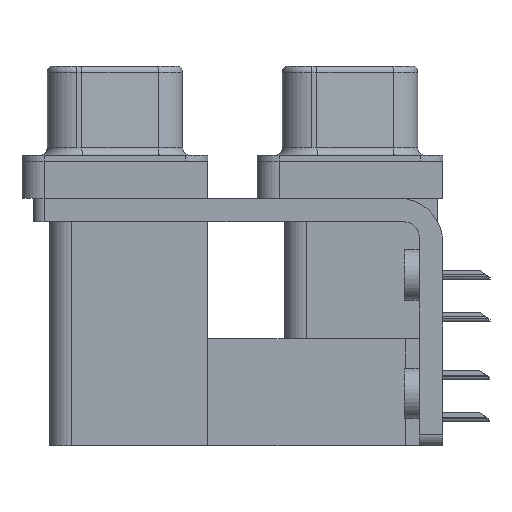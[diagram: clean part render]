
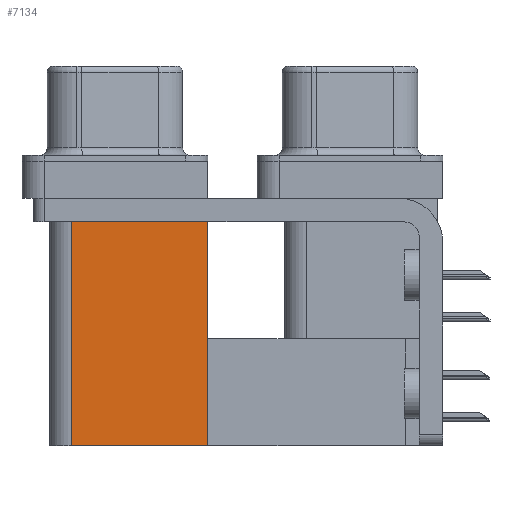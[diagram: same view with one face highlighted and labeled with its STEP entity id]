
A CAD part, left-side view. The second image highlights one B-rep face of the part: STEP entity #7134.
In plain terms, the highlighted planar face has unit normal (-1, 0, 0).
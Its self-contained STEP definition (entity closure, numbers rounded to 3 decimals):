
#318 = EDGE_CURVE ( 'NONE', #9091, #7233, #33261, .T. ) ;
#2637 = CARTESIAN_POINT ( 'NONE',  ( 3.7, 9.6, -2.5 ) ) ;
#3013 = DIRECTION ( 'NONE',  ( 0., 0., 1. ) ) ;
#3194 = EDGE_CURVE ( 'NONE', #9091, #11951, #14326, .T. ) ;
#3592 = DIRECTION ( 'NONE',  ( 0., 1., 0. ) ) ;
#4525 = ORIENTED_EDGE ( 'NONE', *, *, #318, .F. ) ;
#5223 = EDGE_CURVE ( 'NONE', #7233, #37571, #37001, .T. ) ;
#5341 = FACE_OUTER_BOUND ( 'NONE', #20716, .T. ) ;
#6161 = EDGE_CURVE ( 'NONE', #11951, #37571, #36042, .T. ) ;
#6787 = DIRECTION ( 'NONE',  ( 0., 1., 0. ) ) ;
#7134 = ADVANCED_FACE ( 'NONE', ( #5341 ), #27677, .F. ) ;
#7233 = VERTEX_POINT ( 'NONE', #25068 ) ;
#7325 = CARTESIAN_POINT ( 'NONE',  ( 3.7, 18.8, -19.2 ) ) ;
#8796 = DIRECTION ( 'NONE',  ( 0., 0., -1. ) ) ;
#9091 = VERTEX_POINT ( 'NONE', #31145 ) ;
#11951 = VERTEX_POINT ( 'NONE', #2637 ) ;
#12646 = CARTESIAN_POINT ( 'NONE',  ( 3.7, 9.6, -2.5 ) ) ;
#14326 = LINE ( 'NONE', #27563, #18866 ) ;
#15323 = ORIENTED_EDGE ( 'NONE', *, *, #3194, .T. ) ;
#17691 = CARTESIAN_POINT ( 'NONE',  ( 3.7, 18.8, -2.5 ) ) ;
#18103 = DIRECTION ( 'NONE',  ( 1., 0., 0. ) ) ;
#18866 = VECTOR ( 'NONE', #40767, 1000. ) ;
#20716 = EDGE_LOOP ( 'NONE', ( #32661, #38768, #4525, #15323 ) ) ;
#25068 = CARTESIAN_POINT ( 'NONE',  ( 3.7, 18.8, -19.2 ) ) ;
#27563 = CARTESIAN_POINT ( 'NONE',  ( 3.7, 9.6, -19.2 ) ) ;
#27677 = PLANE ( 'NONE',  #33635 ) ;
#29377 = CARTESIAN_POINT ( 'NONE',  ( 3.7, 9.6, -19.2 ) ) ;
#31145 = CARTESIAN_POINT ( 'NONE',  ( 3.7, 9.6, -19.2 ) ) ;
#32133 = VECTOR ( 'NONE', #3013, 1000. ) ;
#32661 = ORIENTED_EDGE ( 'NONE', *, *, #6161, .T. ) ;
#33261 = LINE ( 'NONE', #29377, #36852 ) ;
#33635 = AXIS2_PLACEMENT_3D ( 'NONE', #38485, #18103, #8796 ) ;
#36042 = LINE ( 'NONE', #12646, #37033 ) ;
#36852 = VECTOR ( 'NONE', #3592, 1000. ) ;
#37001 = LINE ( 'NONE', #7325, #32133 ) ;
#37033 = VECTOR ( 'NONE', #6787, 1000. ) ;
#37571 = VERTEX_POINT ( 'NONE', #17691 ) ;
#38485 = CARTESIAN_POINT ( 'NONE',  ( 3.7, 9.6, -19.2 ) ) ;
#38768 = ORIENTED_EDGE ( 'NONE', *, *, #5223, .F. ) ;
#40767 = DIRECTION ( 'NONE',  ( 0., 0., 1. ) ) ;
